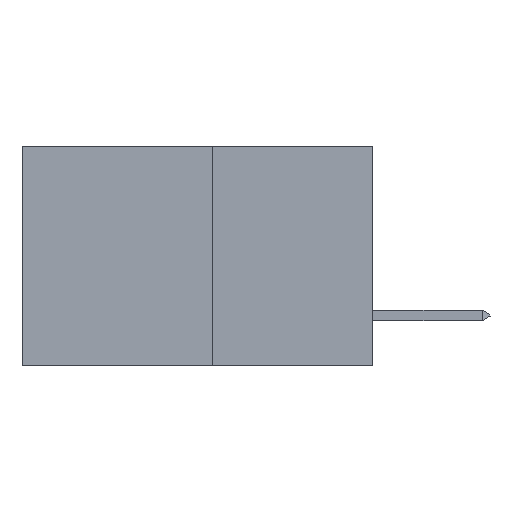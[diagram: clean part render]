
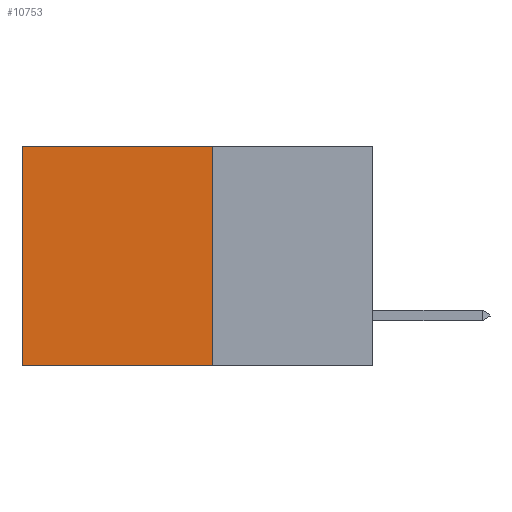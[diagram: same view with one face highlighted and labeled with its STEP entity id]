
A CAD part, left-side view. The second image highlights one B-rep face of the part: STEP entity #10753.
In plain terms, the highlighted planar face has unit normal (-1, 0, 0).
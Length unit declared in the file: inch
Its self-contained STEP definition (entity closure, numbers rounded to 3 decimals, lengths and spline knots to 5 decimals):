
#711 = LINE ( 'NONE', #14141, #15105 ) ;
#1999 = VERTEX_POINT ( 'NONE', #17448 ) ;
#2026 = ORIENTED_EDGE ( 'NONE', *, *, #3465, .F. ) ;
#2901 = FACE_OUTER_BOUND ( 'NONE', #8217, .T. ) ;
#3010 = DIRECTION ( 'NONE',  ( 1., 0., 0. ) ) ;
#3053 = DIRECTION ( 'NONE',  ( 0., 1., 0. ) ) ;
#3465 = EDGE_CURVE ( 'NONE', #13596, #4983, #16497, .T. ) ;
#3517 = CARTESIAN_POINT ( 'NONE',  ( 0.277, 0.27, 0. ) ) ;
#4873 = CARTESIAN_POINT ( 'NONE',  ( 0.277, 0.59, -0.37 ) ) ;
#4983 = VERTEX_POINT ( 'NONE', #4873 ) ;
#6297 = LINE ( 'NONE', #3517, #6760 ) ;
#6760 = VECTOR ( 'NONE', #13324, 39.37008 ) ;
#7227 = CARTESIAN_POINT ( 'NONE',  ( 0.277, 0.27, -0.37 ) ) ;
#7287 = DIRECTION ( 'NONE',  ( 0., 0., -1. ) ) ;
#8217 = EDGE_LOOP ( 'NONE', ( #8636, #2026, #16993, #15283 ) ) ;
#8369 = CARTESIAN_POINT ( 'NONE',  ( 0.277, 0.27, -0.37 ) ) ;
#8636 = ORIENTED_EDGE ( 'NONE', *, *, #14480, .T. ) ;
#8693 = PLANE ( 'NONE',  #16706 ) ;
#9263 = VECTOR ( 'NONE', #14009, 39.37008 ) ;
#10352 = EDGE_CURVE ( 'NONE', #11640, #1999, #6297, .T. ) ;
#10753 = ADVANCED_FACE ( 'NONE', ( #2901 ), #8693, .F. ) ;
#11433 = CARTESIAN_POINT ( 'NONE',  ( 0.277, 0.27, -0.37 ) ) ;
#11640 = VERTEX_POINT ( 'NONE', #13586 ) ;
#12849 = DIRECTION ( 'NONE',  ( 0., 0., -1. ) ) ;
#13238 = EDGE_CURVE ( 'NONE', #11640, #13596, #711, .T. ) ;
#13324 = DIRECTION ( 'NONE',  ( 0., 1., 0. ) ) ;
#13586 = CARTESIAN_POINT ( 'NONE',  ( 0.277, 0.27, 0. ) ) ;
#13596 = VERTEX_POINT ( 'NONE', #8369 ) ;
#14009 = DIRECTION ( 'NONE',  ( 0., 0., -1. ) ) ;
#14141 = CARTESIAN_POINT ( 'NONE',  ( 0.277, 0.27, -0.37 ) ) ;
#14480 = EDGE_CURVE ( 'NONE', #1999, #4983, #16560, .T. ) ;
#15105 = VECTOR ( 'NONE', #7287, 39.37008 ) ;
#15283 = ORIENTED_EDGE ( 'NONE', *, *, #10352, .T. ) ;
#15351 = CARTESIAN_POINT ( 'NONE',  ( 0.277, 0.59, -0.37 ) ) ;
#16086 = VECTOR ( 'NONE', #3053, 39.37008 ) ;
#16497 = LINE ( 'NONE', #7227, #16086 ) ;
#16560 = LINE ( 'NONE', #15351, #9263 ) ;
#16706 = AXIS2_PLACEMENT_3D ( 'NONE', #11433, #3010, #12849 ) ;
#16993 = ORIENTED_EDGE ( 'NONE', *, *, #13238, .F. ) ;
#17448 = CARTESIAN_POINT ( 'NONE',  ( 0.277, 0.59, 0. ) ) ;
